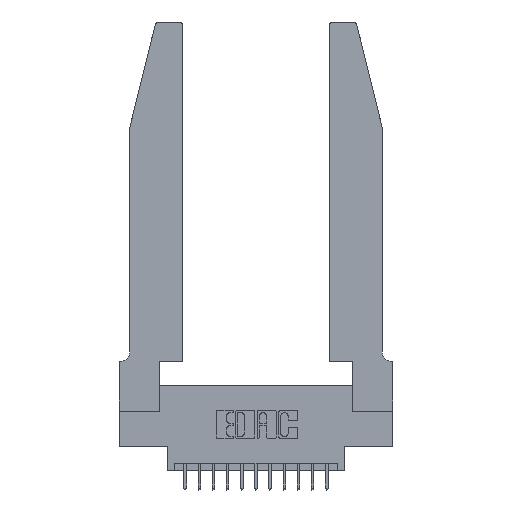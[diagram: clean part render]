
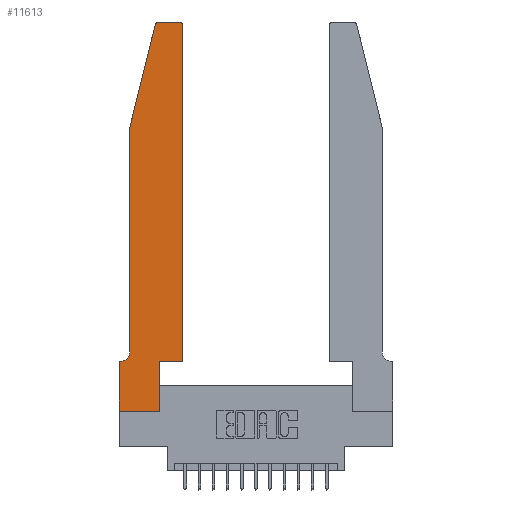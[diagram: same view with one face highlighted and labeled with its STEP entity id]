
A CAD part, top view. The second image highlights one B-rep face of the part: STEP entity #11613.
In plain terms, the highlighted planar face has unit normal (0, 0, 1).
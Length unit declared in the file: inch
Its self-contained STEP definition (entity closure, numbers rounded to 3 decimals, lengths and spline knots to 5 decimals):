
#208 = ORIENTED_EDGE ( 'NONE', *, *, #15056, .T. ) ;
#255 = DIRECTION ( 'NONE',  ( 0., -1., 0. ) ) ;
#567 = FACE_OUTER_BOUND ( 'NONE', #6108, .T. ) ;
#730 = VECTOR ( 'NONE', #12561, 39.37008 ) ;
#931 = DIRECTION ( 'NONE',  ( 0., 0., 1. ) ) ;
#1039 = DIRECTION ( 'NONE',  ( 1., 0., 0. ) ) ;
#1061 = CARTESIAN_POINT ( 'NONE',  ( 0.2605, 2.75, 0.37 ) ) ;
#1380 = VECTOR ( 'NONE', #1039, 39.37008 ) ;
#1603 = VECTOR ( 'NONE', #6427, 39.37008 ) ;
#1609 = CARTESIAN_POINT ( 'NONE',  ( 0.4505, 0.35, 0.37 ) ) ;
#1885 = CARTESIAN_POINT ( 'NONE',  ( 0.0755, 0.35, 0.37 ) ) ;
#1912 = DIRECTION ( 'NONE',  ( 1., 0., 0. ) ) ;
#1990 = VERTEX_POINT ( 'NONE', #17774 ) ;
#2074 = CARTESIAN_POINT ( 'NONE',  ( 0.2865, 0.35, 0.37 ) ) ;
#2292 = CARTESIAN_POINT ( 'NONE',  ( 0., 0., 0.37 ) ) ;
#2313 = ORIENTED_EDGE ( 'NONE', *, *, #12828, .T. ) ;
#2380 = LINE ( 'NONE', #2292, #1380 ) ;
#2920 = VERTEX_POINT ( 'NONE', #8143 ) ;
#3248 = LINE ( 'NONE', #11759, #1603 ) ;
#3808 = EDGE_CURVE ( 'NONE', #9293, #1990, #12169, .T. ) ;
#4180 = ORIENTED_EDGE ( 'NONE', *, *, #11402, .T. ) ;
#4263 = DIRECTION ( 'NONE',  ( 0., -1., 0. ) ) ;
#4400 = ORIENTED_EDGE ( 'NONE', *, *, #15163, .T. ) ;
#4513 = ORIENTED_EDGE ( 'NONE', *, *, #6692, .T. ) ;
#4718 = VERTEX_POINT ( 'NONE', #14007 ) ;
#4815 = ORIENTED_EDGE ( 'NONE', *, *, #12316, .T. ) ;
#4878 = DIRECTION ( 'NONE',  ( 0., 1., 0. ) ) ;
#4897 = LINE ( 'NONE', #14922, #5954 ) ;
#5053 = VECTOR ( 'NONE', #4878, 39.37008 ) ;
#5531 = VERTEX_POINT ( 'NONE', #15956 ) ;
#5534 = DIRECTION ( 'NONE',  ( 0., 1., 0. ) ) ;
#5954 = VECTOR ( 'NONE', #5534, 39.37008 ) ;
#6108 = EDGE_LOOP ( 'NONE', ( #10372, #208, #4815, #4180, #8889, #7726, #7603, #2313, #13037, #4400, #12673, #4513 ) ) ;
#6427 = DIRECTION ( 'NONE',  ( -0.239, -0.971, 0. ) ) ;
#6692 = EDGE_CURVE ( 'NONE', #7481, #9293, #17636, .T. ) ;
#6743 = CARTESIAN_POINT ( 'NONE',  ( 0.4505, 2.72, 0.37 ) ) ;
#7113 = LINE ( 'NONE', #11177, #17690 ) ;
#7161 = VERTEX_POINT ( 'NONE', #12012 ) ;
#7481 = VERTEX_POINT ( 'NONE', #6743 ) ;
#7603 = ORIENTED_EDGE ( 'NONE', *, *, #14027, .T. ) ;
#7726 = ORIENTED_EDGE ( 'NONE', *, *, #9365, .T. ) ;
#8143 = CARTESIAN_POINT ( 'NONE',  ( 0.0755, 0.42, 0.37 ) ) ;
#8370 = LINE ( 'NONE', #13870, #14614 ) ;
#8597 = PLANE ( 'NONE',  #16334 ) ;
#8777 = CARTESIAN_POINT ( 'NONE',  ( 0.25487, 2.72718, 0.37 ) ) ;
#8889 = ORIENTED_EDGE ( 'NONE', *, *, #14135, .T. ) ;
#8945 = CARTESIAN_POINT ( 'NONE',  ( 0.2865, 0., 0.37 ) ) ;
#8969 = DIRECTION ( 'NONE',  ( 1., 0., 0. ) ) ;
#9293 = VERTEX_POINT ( 'NONE', #16790 ) ;
#9365 = EDGE_CURVE ( 'NONE', #5531, #17679, #15421, .T. ) ;
#9598 = EDGE_CURVE ( 'NONE', #13573, #7161, #14537, .T. ) ;
#9605 = AXIS2_PLACEMENT_3D ( 'NONE', #15380, #17003, #16913 ) ;
#9670 = VERTEX_POINT ( 'NONE', #8777 ) ;
#9925 = DIRECTION ( 'NONE',  ( 1., 0., 0. ) ) ;
#10037 = CARTESIAN_POINT ( 'NONE',  ( 0., 0., 0.37 ) ) ;
#10372 = ORIENTED_EDGE ( 'NONE', *, *, #3808, .T. ) ;
#10548 = DIRECTION ( 'NONE',  ( -1., 0., 0. ) ) ;
#10806 = EDGE_CURVE ( 'NONE', #4718, #7481, #4897, .T. ) ;
#11177 = CARTESIAN_POINT ( 'NONE',  ( 0., 0., 0.37 ) ) ;
#11402 = EDGE_CURVE ( 'NONE', #12979, #2920, #8370, .T. ) ;
#11591 = CARTESIAN_POINT ( 'NONE',  ( 0., 0.35, 0.37 ) ) ;
#11613 = ADVANCED_FACE ( 'NONE', ( #567 ), #8597, .T. ) ;
#11732 = VECTOR ( 'NONE', #9925, 39.37008 ) ;
#11759 = CARTESIAN_POINT ( 'NONE',  ( 0.0755, 2., 0.37 ) ) ;
#12012 = CARTESIAN_POINT ( 'NONE',  ( 0.2865, 0.35, 0.37 ) ) ;
#12169 = LINE ( 'NONE', #1061, #17344 ) ;
#12177 = VERTEX_POINT ( 'NONE', #10037 ) ;
#12316 = EDGE_CURVE ( 'NONE', #9670, #12979, #3248, .T. ) ;
#12375 = LINE ( 'NONE', #1609, #11732 ) ;
#12561 = DIRECTION ( 'NONE',  ( -1., 0., 0. ) ) ;
#12580 = AXIS2_PLACEMENT_3D ( 'NONE', #16073, #931, #8969 ) ;
#12673 = ORIENTED_EDGE ( 'NONE', *, *, #10806, .T. ) ;
#12828 = EDGE_CURVE ( 'NONE', #12177, #13573, #2380, .T. ) ;
#12979 = VERTEX_POINT ( 'NONE', #17146 ) ;
#13037 = ORIENTED_EDGE ( 'NONE', *, *, #9598, .T. ) ;
#13573 = VERTEX_POINT ( 'NONE', #8945 ) ;
#13870 = CARTESIAN_POINT ( 'NONE',  ( 0.0755, 2., 0.37 ) ) ;
#13985 = CIRCLE ( 'NONE', #14554, 0.07 ) ;
#14007 = CARTESIAN_POINT ( 'NONE',  ( 0.4505, 0.35, 0.37 ) ) ;
#14027 = EDGE_CURVE ( 'NONE', #17679, #12177, #7113, .T. ) ;
#14135 = EDGE_CURVE ( 'NONE', #2920, #5531, #13985, .T. ) ;
#14537 = LINE ( 'NONE', #2074, #5053 ) ;
#14551 = DIRECTION ( 'NONE',  ( 0., 0., -1. ) ) ;
#14554 = AXIS2_PLACEMENT_3D ( 'NONE', #16755, #14551, #17083 ) ;
#14614 = VECTOR ( 'NONE', #4263, 39.37008 ) ;
#14922 = CARTESIAN_POINT ( 'NONE',  ( 0.4505, 0.35, 0.37 ) ) ;
#15056 = EDGE_CURVE ( 'NONE', #1990, #9670, #15156, .T. ) ;
#15156 = CIRCLE ( 'NONE', #12580, 0.03 ) ;
#15163 = EDGE_CURVE ( 'NONE', #7161, #4718, #12375, .T. ) ;
#15380 = CARTESIAN_POINT ( 'NONE',  ( 0.4205, 2.72, 0.37 ) ) ;
#15421 = LINE ( 'NONE', #1885, #730 ) ;
#15956 = CARTESIAN_POINT ( 'NONE',  ( 0.0055, 0.35, 0.37 ) ) ;
#16073 = CARTESIAN_POINT ( 'NONE',  ( 0.284, 2.72, 0.37 ) ) ;
#16334 = AXIS2_PLACEMENT_3D ( 'NONE', #11591, #16892, #1912 ) ;
#16755 = CARTESIAN_POINT ( 'NONE',  ( 0.0055, 0.42, 0.37 ) ) ;
#16790 = CARTESIAN_POINT ( 'NONE',  ( 0.4205, 2.75, 0.37 ) ) ;
#16794 = CARTESIAN_POINT ( 'NONE',  ( 0., 0.35, 0.37 ) ) ;
#16892 = DIRECTION ( 'NONE',  ( 0., 0., 1. ) ) ;
#16913 = DIRECTION ( 'NONE',  ( 1., 0., 0. ) ) ;
#17003 = DIRECTION ( 'NONE',  ( 0., 0., 1. ) ) ;
#17083 = DIRECTION ( 'NONE',  ( -1., 0., 0. ) ) ;
#17146 = CARTESIAN_POINT ( 'NONE',  ( 0.0755, 2., 0.37 ) ) ;
#17344 = VECTOR ( 'NONE', #10548, 39.37008 ) ;
#17636 = CIRCLE ( 'NONE', #9605, 0.03 ) ;
#17679 = VERTEX_POINT ( 'NONE', #16794 ) ;
#17690 = VECTOR ( 'NONE', #255, 39.37008 ) ;
#17774 = CARTESIAN_POINT ( 'NONE',  ( 0.284, 2.75, 0.37 ) ) ;
